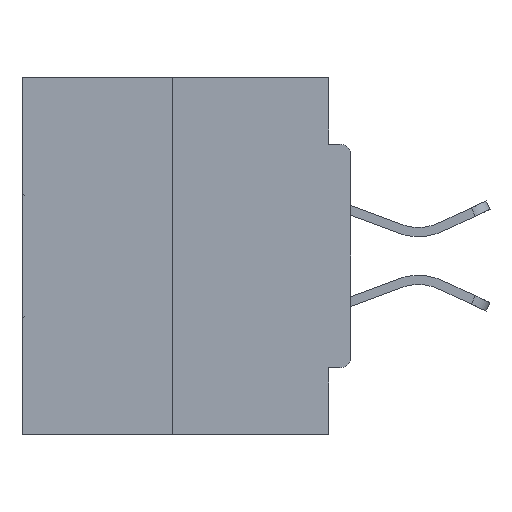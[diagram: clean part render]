
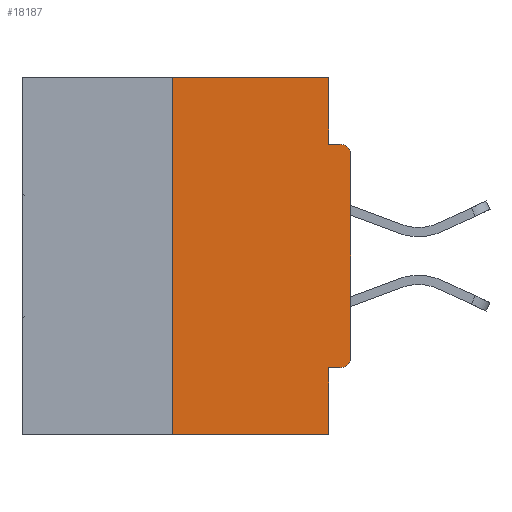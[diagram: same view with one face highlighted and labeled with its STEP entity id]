
A CAD part, left-side view. The second image highlights one B-rep face of the part: STEP entity #18187.
In plain terms, the highlighted planar face has unit normal (-1, 0, 0).
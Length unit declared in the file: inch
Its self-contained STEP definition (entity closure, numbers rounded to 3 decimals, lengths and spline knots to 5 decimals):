
#210 = DIRECTION ( 'NONE',  ( 0., 0., 1. ) ) ;
#324 = CARTESIAN_POINT ( 'NONE',  ( 0., 0.031, -0.0935 ) ) ;
#589 = CARTESIAN_POINT ( 'NONE',  ( 0., 0.46, 0. ) ) ;
#852 = DIRECTION ( 'NONE',  ( 1., 0., 0. ) ) ;
#1068 = VERTEX_POINT ( 'NONE', #22257 ) ;
#1137 = CARTESIAN_POINT ( 'NONE',  ( 0., 0., -0.3915 ) ) ;
#1548 = CARTESIAN_POINT ( 'NONE',  ( 0., 0.46, -0.5 ) ) ;
#2364 = LINE ( 'NONE', #21980, #14769 ) ;
#2677 = EDGE_LOOP ( 'NONE', ( #26055, #3402, #13287, #20363, #30167, #38337, #22097, #37969, #39646, #17416 ) ) ;
#3402 = ORIENTED_EDGE ( 'NONE', *, *, #20738, .F. ) ;
#3475 = DIRECTION ( 'NONE',  ( 0., 0., -1. ) ) ;
#3735 = VECTOR ( 'NONE', #22120, 39.37008 ) ;
#4487 = CARTESIAN_POINT ( 'NONE',  ( 0., 0.015, -0.3915 ) ) ;
#4577 = CARTESIAN_POINT ( 'NONE',  ( 0., 0.015, -0.4065 ) ) ;
#4619 = DIRECTION ( 'NONE',  ( 0., 0., -1. ) ) ;
#4693 = VECTOR ( 'NONE', #37216, 39.37008 ) ;
#4706 = CARTESIAN_POINT ( 'NONE',  ( 0., 0.015, -0.1085 ) ) ;
#4991 = CARTESIAN_POINT ( 'NONE',  ( 0., 0., 0. ) ) ;
#6051 = VERTEX_POINT ( 'NONE', #324 ) ;
#7044 = VERTEX_POINT ( 'NONE', #1137 ) ;
#7095 = EDGE_CURVE ( 'NONE', #31845, #17084, #24729, .T. ) ;
#7226 = EDGE_CURVE ( 'NONE', #32692, #7044, #32714, .T. ) ;
#8109 = DIRECTION ( 'NONE',  ( 0., 0., -1. ) ) ;
#8436 = EDGE_CURVE ( 'NONE', #1068, #39772, #23166, .T. ) ;
#8447 = DIRECTION ( 'NONE',  ( 0., 0., -1. ) ) ;
#8692 = LINE ( 'NONE', #15334, #3735 ) ;
#8739 = VECTOR ( 'NONE', #16340, 39.37008 ) ;
#9606 = LINE ( 'NONE', #17919, #31917 ) ;
#10267 = PLANE ( 'NONE',  #28076 ) ;
#10621 = AXIS2_PLACEMENT_3D ( 'NONE', #4706, #21047, #8447 ) ;
#13287 = ORIENTED_EDGE ( 'NONE', *, *, #34798, .T. ) ;
#13609 = VECTOR ( 'NONE', #15094, 39.37008 ) ;
#14769 = VECTOR ( 'NONE', #40505, 39.37008 ) ;
#15094 = DIRECTION ( 'NONE',  ( 0., 0., 1. ) ) ;
#15197 = CARTESIAN_POINT ( 'NONE',  ( 0., 0.015, -0.0935 ) ) ;
#15334 = CARTESIAN_POINT ( 'NONE',  ( 0., 0., -0.0935 ) ) ;
#15762 = CARTESIAN_POINT ( 'NONE',  ( 0., 0.031, 0. ) ) ;
#16340 = DIRECTION ( 'NONE',  ( 0., -1., 0. ) ) ;
#16367 = CARTESIAN_POINT ( 'NONE',  ( 0., 0.031, -0.5 ) ) ;
#16935 = VECTOR ( 'NONE', #3475, 39.37008 ) ;
#17084 = VERTEX_POINT ( 'NONE', #15197 ) ;
#17300 = CARTESIAN_POINT ( 'NONE',  ( 0., 0.031, -0.4065 ) ) ;
#17416 = ORIENTED_EDGE ( 'NONE', *, *, #24793, .F. ) ;
#17919 = CARTESIAN_POINT ( 'NONE',  ( 0., 0.031, 0. ) ) ;
#18187 = ADVANCED_FACE ( 'NONE', ( #28511 ), #10267, .F. ) ;
#18485 = EDGE_CURVE ( 'NONE', #6051, #17084, #8692, .T. ) ;
#20363 = ORIENTED_EDGE ( 'NONE', *, *, #31016, .F. ) ;
#20738 = EDGE_CURVE ( 'NONE', #34059, #1068, #32394, .T. ) ;
#21047 = DIRECTION ( 'NONE',  ( -1., 0., 0. ) ) ;
#21980 = CARTESIAN_POINT ( 'NONE',  ( 0., 0., -0.4065 ) ) ;
#22097 = ORIENTED_EDGE ( 'NONE', *, *, #40679, .T. ) ;
#22120 = DIRECTION ( 'NONE',  ( 0., -1., 0. ) ) ;
#22257 = CARTESIAN_POINT ( 'NONE',  ( 0., 0.25, 0. ) ) ;
#23166 = LINE ( 'NONE', #26298, #8739 ) ;
#24729 = CIRCLE ( 'NONE', #10621, 0.015 ) ;
#24793 = EDGE_CURVE ( 'NONE', #39772, #6051, #9606, .T. ) ;
#26055 = ORIENTED_EDGE ( 'NONE', *, *, #8436, .F. ) ;
#26298 = CARTESIAN_POINT ( 'NONE',  ( 0., 0.46, 0. ) ) ;
#27726 = CARTESIAN_POINT ( 'NONE',  ( 0., 0., -0.1085 ) ) ;
#28076 = AXIS2_PLACEMENT_3D ( 'NONE', #589, #852, #38723 ) ;
#28511 = FACE_OUTER_BOUND ( 'NONE', #2677, .T. ) ;
#29977 = LINE ( 'NONE', #4991, #13609 ) ;
#30167 = ORIENTED_EDGE ( 'NONE', *, *, #37755, .F. ) ;
#31016 = EDGE_CURVE ( 'NONE', #35002, #36427, #40788, .T. ) ;
#31845 = VERTEX_POINT ( 'NONE', #27726 ) ;
#31917 = VECTOR ( 'NONE', #8109, 39.37008 ) ;
#32394 = LINE ( 'NONE', #38210, #39863 ) ;
#32692 = VERTEX_POINT ( 'NONE', #4577 ) ;
#32714 = CIRCLE ( 'NONE', #39056, 0.015 ) ;
#34059 = VERTEX_POINT ( 'NONE', #39774 ) ;
#34798 = EDGE_CURVE ( 'NONE', #34059, #36427, #39959, .T. ) ;
#35002 = VERTEX_POINT ( 'NONE', #17300 ) ;
#35654 = CARTESIAN_POINT ( 'NONE',  ( 0., 0.031, -0.5 ) ) ;
#36427 = VERTEX_POINT ( 'NONE', #35654 ) ;
#36670 = DIRECTION ( 'NONE',  ( -1., 0., 0. ) ) ;
#37216 = DIRECTION ( 'NONE',  ( 0., -1., 0. ) ) ;
#37755 = EDGE_CURVE ( 'NONE', #32692, #35002, #2364, .T. ) ;
#37969 = ORIENTED_EDGE ( 'NONE', *, *, #7095, .T. ) ;
#38210 = CARTESIAN_POINT ( 'NONE',  ( 0., 0.25, 0. ) ) ;
#38337 = ORIENTED_EDGE ( 'NONE', *, *, #7226, .T. ) ;
#38723 = DIRECTION ( 'NONE',  ( 0., 0., -1. ) ) ;
#39056 = AXIS2_PLACEMENT_3D ( 'NONE', #4487, #36670, #4619 ) ;
#39646 = ORIENTED_EDGE ( 'NONE', *, *, #18485, .F. ) ;
#39772 = VERTEX_POINT ( 'NONE', #15762 ) ;
#39774 = CARTESIAN_POINT ( 'NONE',  ( 0., 0.25, -0.5 ) ) ;
#39863 = VECTOR ( 'NONE', #210, 39.37008 ) ;
#39959 = LINE ( 'NONE', #1548, #4693 ) ;
#40505 = DIRECTION ( 'NONE',  ( 0., 1., 0. ) ) ;
#40679 = EDGE_CURVE ( 'NONE', #7044, #31845, #29977, .T. ) ;
#40788 = LINE ( 'NONE', #16367, #16935 ) ;
